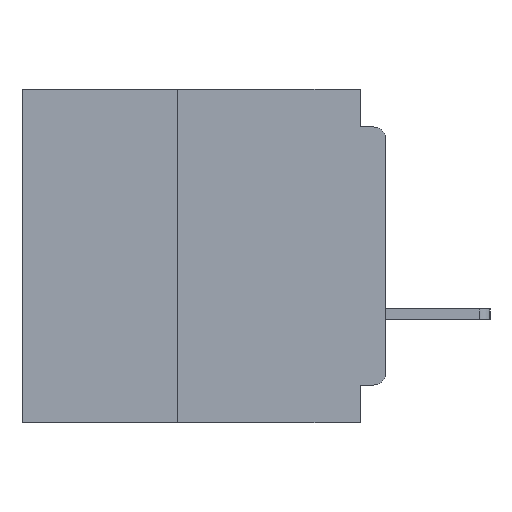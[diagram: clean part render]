
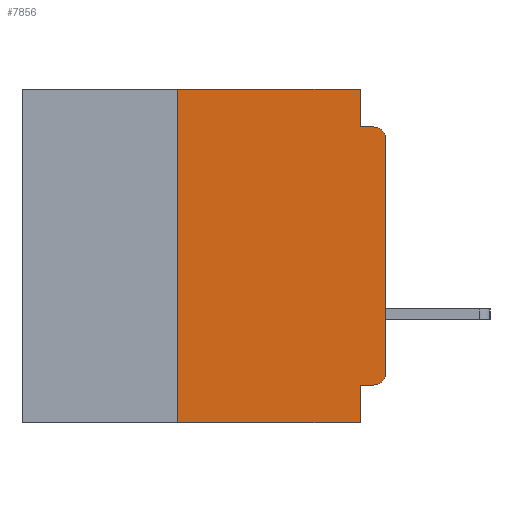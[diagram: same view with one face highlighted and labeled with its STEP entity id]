
A CAD part, left-side view. The second image highlights one B-rep face of the part: STEP entity #7856.
In plain terms, the highlighted planar face has unit normal (-1, 0, 0).
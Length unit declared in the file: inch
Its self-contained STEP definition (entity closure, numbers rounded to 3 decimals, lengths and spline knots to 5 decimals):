
#76 = ORIENTED_EDGE ( 'NONE', *, *, #12543, .F. ) ;
#298 = FACE_OUTER_BOUND ( 'NONE', #23753, .T. ) ;
#557 = VERTEX_POINT ( 'NONE', #35537 ) ;
#2021 = DIRECTION ( 'NONE',  ( -1., 0., 0. ) ) ;
#4257 = VERTEX_POINT ( 'NONE', #13889 ) ;
#5100 = CIRCLE ( 'NONE', #22772, 0.015 ) ;
#5742 = VECTOR ( 'NONE', #8936, 39.37008 ) ;
#5969 = CARTESIAN_POINT ( 'NONE',  ( 0., 0., 0. ) ) ;
#6656 = EDGE_CURVE ( 'NONE', #15235, #23024, #8876, .T. ) ;
#6812 = LINE ( 'NONE', #29070, #5742 ) ;
#7025 = CARTESIAN_POINT ( 'NONE',  ( 0., 0., -0.355 ) ) ;
#7856 = ADVANCED_FACE ( 'NONE', ( #298 ), #38792, .F. ) ;
#8623 = VERTEX_POINT ( 'NONE', #39724 ) ;
#8876 = LINE ( 'NONE', #29478, #34519 ) ;
#8936 = DIRECTION ( 'NONE',  ( 0., 0., -1. ) ) ;
#10478 = LINE ( 'NONE', #5969, #30402 ) ;
#11127 = DIRECTION ( 'NONE',  ( 0., 0., 1. ) ) ;
#11851 = VERTEX_POINT ( 'NONE', #14272 ) ;
#11854 = CARTESIAN_POINT ( 'NONE',  ( 0., 0.031, -0.355 ) ) ;
#12543 = EDGE_CURVE ( 'NONE', #557, #27942, #20182, .T. ) ;
#13338 = VERTEX_POINT ( 'NONE', #22344 ) ;
#13889 = CARTESIAN_POINT ( 'NONE',  ( 0., 0., -0.06 ) ) ;
#14234 = CARTESIAN_POINT ( 'NONE',  ( 0., 0.015, -0.06 ) ) ;
#14272 = CARTESIAN_POINT ( 'NONE',  ( 0., 0.015, -0.355 ) ) ;
#14327 = CARTESIAN_POINT ( 'NONE',  ( 0., 0.25, -0.4 ) ) ;
#14699 = AXIS2_PLACEMENT_3D ( 'NONE', #22224, #2021, #25589 ) ;
#15235 = VERTEX_POINT ( 'NONE', #16078 ) ;
#15696 = CARTESIAN_POINT ( 'NONE',  ( 0., 0.031, 0. ) ) ;
#15801 = EDGE_CURVE ( 'NONE', #21520, #23024, #6812, .T. ) ;
#15989 = CARTESIAN_POINT ( 'NONE',  ( 0., 0., -0.045 ) ) ;
#16078 = CARTESIAN_POINT ( 'NONE',  ( 0., 0.25, -0.4 ) ) ;
#16697 = EDGE_CURVE ( 'NONE', #13338, #4257, #10478, .T. ) ;
#17323 = EDGE_CURVE ( 'NONE', #23179, #8623, #40593, .T. ) ;
#17391 = ORIENTED_EDGE ( 'NONE', *, *, #29494, .T. ) ;
#17475 = ORIENTED_EDGE ( 'NONE', *, *, #17323, .F. ) ;
#17618 = DIRECTION ( 'NONE',  ( 0., 0., -1. ) ) ;
#17637 = LINE ( 'NONE', #29781, #43043 ) ;
#18047 = CARTESIAN_POINT ( 'NONE',  ( 0., 0.437, 0. ) ) ;
#18697 = EDGE_CURVE ( 'NONE', #27942, #23179, #17637, .T. ) ;
#19175 = CARTESIAN_POINT ( 'NONE',  ( 0., 0.031, -0.045 ) ) ;
#19211 = DIRECTION ( 'NONE',  ( 1., 0., 0. ) ) ;
#19356 = DIRECTION ( 'NONE',  ( 0., -1., 0. ) ) ;
#20182 = LINE ( 'NONE', #18047, #30130 ) ;
#20914 = VECTOR ( 'NONE', #19356, 39.37008 ) ;
#21520 = VERTEX_POINT ( 'NONE', #11854 ) ;
#21881 = VECTOR ( 'NONE', #27166, 39.37008 ) ;
#22190 = ORIENTED_EDGE ( 'NONE', *, *, #18697, .F. ) ;
#22224 = CARTESIAN_POINT ( 'NONE',  ( 0., 0.015, -0.34 ) ) ;
#22344 = CARTESIAN_POINT ( 'NONE',  ( 0., 0., -0.34 ) ) ;
#22772 = AXIS2_PLACEMENT_3D ( 'NONE', #14234, #37521, #17618 ) ;
#23024 = VERTEX_POINT ( 'NONE', #38337 ) ;
#23092 = LINE ( 'NONE', #14327, #39651 ) ;
#23179 = VERTEX_POINT ( 'NONE', #19175 ) ;
#23753 = EDGE_LOOP ( 'NONE', ( #25671, #17391, #17475, #22190, #76, #37557, #37621, #38817, #32038, #31969 ) ) ;
#25589 = DIRECTION ( 'NONE',  ( 0., 0., -1. ) ) ;
#25671 = ORIENTED_EDGE ( 'NONE', *, *, #16697, .T. ) ;
#25784 = CARTESIAN_POINT ( 'NONE',  ( 0., 0.437, 0. ) ) ;
#27166 = DIRECTION ( 'NONE',  ( 0., 1., 0. ) ) ;
#27942 = VERTEX_POINT ( 'NONE', #15696 ) ;
#29070 = CARTESIAN_POINT ( 'NONE',  ( 0., 0.031, -0.4 ) ) ;
#29478 = CARTESIAN_POINT ( 'NONE',  ( 0., 0.437, -0.4 ) ) ;
#29494 = EDGE_CURVE ( 'NONE', #4257, #8623, #5100, .T. ) ;
#29513 = DIRECTION ( 'NONE',  ( 0., 0., 1. ) ) ;
#29781 = CARTESIAN_POINT ( 'NONE',  ( 0., 0.031, 0. ) ) ;
#30130 = VECTOR ( 'NONE', #31348, 39.37008 ) ;
#30402 = VECTOR ( 'NONE', #29513, 39.37008 ) ;
#31348 = DIRECTION ( 'NONE',  ( 0., -1., 0. ) ) ;
#31631 = EDGE_CURVE ( 'NONE', #11851, #13338, #40409, .T. ) ;
#31969 = ORIENTED_EDGE ( 'NONE', *, *, #31631, .T. ) ;
#32038 = ORIENTED_EDGE ( 'NONE', *, *, #41431, .F. ) ;
#34519 = VECTOR ( 'NONE', #42690, 39.37008 ) ;
#35537 = CARTESIAN_POINT ( 'NONE',  ( 0., 0.25, 0. ) ) ;
#36564 = EDGE_CURVE ( 'NONE', #15235, #557, #23092, .T. ) ;
#37521 = DIRECTION ( 'NONE',  ( -1., 0., 0. ) ) ;
#37557 = ORIENTED_EDGE ( 'NONE', *, *, #36564, .F. ) ;
#37621 = ORIENTED_EDGE ( 'NONE', *, *, #6656, .T. ) ;
#38337 = CARTESIAN_POINT ( 'NONE',  ( 0., 0.031, -0.4 ) ) ;
#38792 = PLANE ( 'NONE',  #42966 ) ;
#38817 = ORIENTED_EDGE ( 'NONE', *, *, #15801, .F. ) ;
#39490 = LINE ( 'NONE', #7025, #21881 ) ;
#39651 = VECTOR ( 'NONE', #11127, 39.37008 ) ;
#39673 = DIRECTION ( 'NONE',  ( 0., 0., -1. ) ) ;
#39724 = CARTESIAN_POINT ( 'NONE',  ( 0., 0.015, -0.045 ) ) ;
#40409 = CIRCLE ( 'NONE', #14699, 0.015 ) ;
#40593 = LINE ( 'NONE', #15989, #20914 ) ;
#41431 = EDGE_CURVE ( 'NONE', #11851, #21520, #39490, .T. ) ;
#42379 = DIRECTION ( 'NONE',  ( 0., 0., -1. ) ) ;
#42690 = DIRECTION ( 'NONE',  ( 0., -1., 0. ) ) ;
#42966 = AXIS2_PLACEMENT_3D ( 'NONE', #25784, #19211, #42379 ) ;
#43043 = VECTOR ( 'NONE', #39673, 39.37008 ) ;
